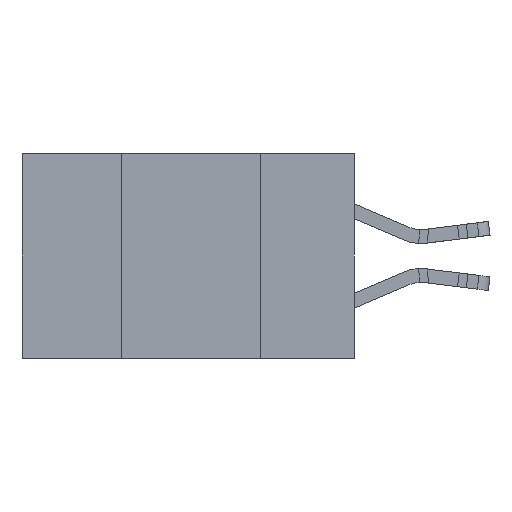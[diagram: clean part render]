
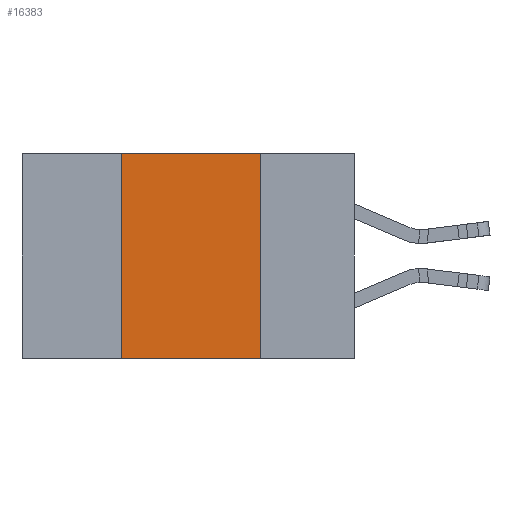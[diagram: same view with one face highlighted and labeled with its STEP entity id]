
A CAD part, left-side view. The second image highlights one B-rep face of the part: STEP entity #16383.
In plain terms, the highlighted planar face has unit normal (-1, 0, 0).
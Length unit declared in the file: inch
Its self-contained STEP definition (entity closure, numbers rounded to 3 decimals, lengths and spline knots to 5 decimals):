
#693 = EDGE_CURVE ( 'NONE', #4287, #17642, #13874, .T. ) ;
#1008 = FACE_OUTER_BOUND ( 'NONE', #3532, .T. ) ;
#3322 = CARTESIAN_POINT ( 'NONE',  ( 0., 0.42, 0. ) ) ;
#3532 = EDGE_LOOP ( 'NONE', ( #24953, #19997, #19505, #4725 ) ) ;
#3793 = CARTESIAN_POINT ( 'NONE',  ( 0., 0.17, -0.37 ) ) ;
#3921 = EDGE_CURVE ( 'NONE', #25821, #17642, #13353, .T. ) ;
#4287 = VERTEX_POINT ( 'NONE', #20586 ) ;
#4597 = DIRECTION ( 'NONE',  ( 1., 0., 0. ) ) ;
#4725 = ORIENTED_EDGE ( 'NONE', *, *, #3921, .T. ) ;
#7470 = CARTESIAN_POINT ( 'NONE',  ( 0., 0.6, 0. ) ) ;
#7566 = VECTOR ( 'NONE', #7906, 39.37008 ) ;
#7906 = DIRECTION ( 'NONE',  ( 0., 0., -1. ) ) ;
#10160 = VECTOR ( 'NONE', #21648, 39.37008 ) ;
#11273 = CARTESIAN_POINT ( 'NONE',  ( 0., 0.42, -0.37 ) ) ;
#12277 = CARTESIAN_POINT ( 'NONE',  ( 0., 0.17, -0.37 ) ) ;
#12473 = EDGE_CURVE ( 'NONE', #25821, #18854, #15761, .T. ) ;
#12676 = CARTESIAN_POINT ( 'NONE',  ( 0., 0.6, 0. ) ) ;
#13238 = EDGE_CURVE ( 'NONE', #18854, #4287, #15559, .T. ) ;
#13353 = LINE ( 'NONE', #23540, #14182 ) ;
#13734 = CARTESIAN_POINT ( 'NONE',  ( 0., 0.42, -0.37 ) ) ;
#13874 = LINE ( 'NONE', #12277, #7566 ) ;
#14182 = VECTOR ( 'NONE', #23015, 39.37008 ) ;
#15371 = DIRECTION ( 'NONE',  ( 0., 0., 1. ) ) ;
#15559 = LINE ( 'NONE', #7470, #10160 ) ;
#15761 = LINE ( 'NONE', #11273, #20302 ) ;
#16383 = ADVANCED_FACE ( 'NONE', ( #1008 ), #20749, .F. ) ;
#17642 = VERTEX_POINT ( 'NONE', #3793 ) ;
#18854 = VERTEX_POINT ( 'NONE', #3322 ) ;
#19505 = ORIENTED_EDGE ( 'NONE', *, *, #12473, .F. ) ;
#19997 = ORIENTED_EDGE ( 'NONE', *, *, #13238, .F. ) ;
#20302 = VECTOR ( 'NONE', #15371, 39.37008 ) ;
#20586 = CARTESIAN_POINT ( 'NONE',  ( 0., 0.17, 0. ) ) ;
#20749 = PLANE ( 'NONE',  #24396 ) ;
#21009 = DIRECTION ( 'NONE',  ( 0., 0., -1. ) ) ;
#21648 = DIRECTION ( 'NONE',  ( 0., -1., 0. ) ) ;
#23015 = DIRECTION ( 'NONE',  ( 0., -1., 0. ) ) ;
#23540 = CARTESIAN_POINT ( 'NONE',  ( 0., 0.6, -0.37 ) ) ;
#24396 = AXIS2_PLACEMENT_3D ( 'NONE', #12676, #4597, #21009 ) ;
#24953 = ORIENTED_EDGE ( 'NONE', *, *, #693, .F. ) ;
#25821 = VERTEX_POINT ( 'NONE', #13734 ) ;
